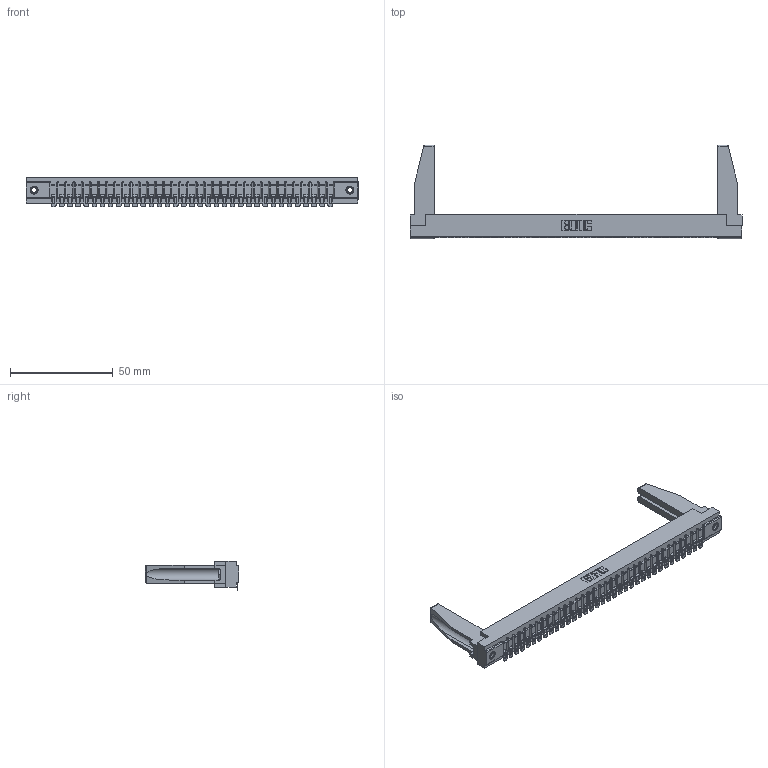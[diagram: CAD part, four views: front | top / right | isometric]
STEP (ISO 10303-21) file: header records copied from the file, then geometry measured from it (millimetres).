
FILE_DESCRIPTION (( 'STEP AP203' ), '1' );
FILE_NAME ('357-035-454-178.STEP', '2020-10-02T15:55:08', ( '' ), ( '' ), 'SwSTEP 2.0', 'SolidWorks 2020', '' );
FILE_SCHEMA (( 'CONFIG_CONTROL_DESIGN' ));
Length unit declared in the file: inch
Products named in the file (5): 307-220-078; 307 Part_.156 Dia Mounting Holes; 345-250-001_345-250-001-102; 357-035-454-178; 307-290-002_554
Assembly tree (40 placements, depth 2):
  357-035-454-178
    307 Part_.156 Dia Mounting Holes
    307-290-002_554  x35
    307-220-078  x2
    345-250-001_345-250-001-102  x2
Bounding box: 161.7 x 45.72 x 14.52 mm (x, y, z)
Volume: 21257.3 mm3; surface area: 25513.9 mm2
Topology: 40 solids, 40 shells, 3119 faces, 9508 edges, 6232 vertices
Faces by surface type: plane 1764, cylinder 1267, sphere 72, cone 12, torus 4
Entity records: 34272 total; most frequent: CARTESIAN_POINT 5780, ORIENTED_EDGE 5726, DIRECTION 5581, EDGE_CURVE 2863, LINE 2187, VECTOR 2187, VERTEX_POINT 1854, AXIS2_PLACEMENT_3D 1697
